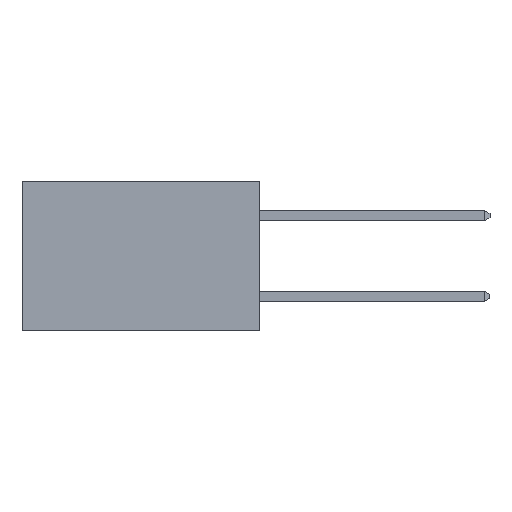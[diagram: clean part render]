
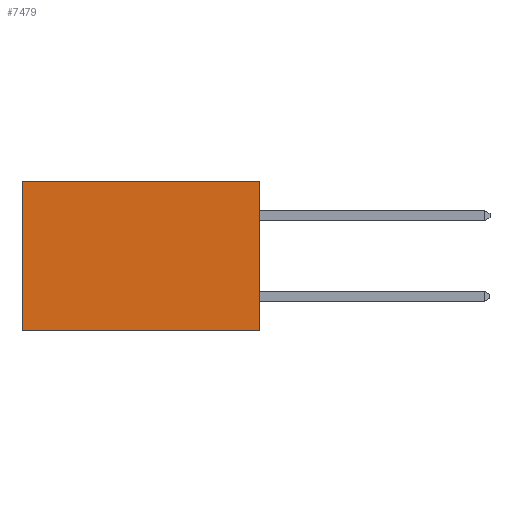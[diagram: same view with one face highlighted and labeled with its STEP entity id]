
A CAD part, left-side view. The second image highlights one B-rep face of the part: STEP entity #7479.
In plain terms, the highlighted planar face has unit normal (-1, 0, 0).
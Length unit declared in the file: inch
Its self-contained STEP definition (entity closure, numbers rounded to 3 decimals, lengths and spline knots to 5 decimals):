
#136 = CARTESIAN_POINT ( 'NONE',  ( 0.277, 0., 0. ) ) ;
#254 = EDGE_LOOP ( 'NONE', ( #7141, #4516, #5979, #3361 ) ) ;
#723 = LINE ( 'NONE', #136, #1090 ) ;
#1090 = VECTOR ( 'NONE', #7407, 39.37008 ) ;
#1256 = CARTESIAN_POINT ( 'NONE',  ( 0.277, 0.59, -0.37 ) ) ;
#1434 = CARTESIAN_POINT ( 'NONE',  ( 0.277, 0., -0.37 ) ) ;
#1784 = DIRECTION ( 'NONE',  ( 0., 0., -1. ) ) ;
#1935 = DIRECTION ( 'NONE',  ( 0., 0., -1. ) ) ;
#1947 = DIRECTION ( 'NONE',  ( 1., 0., 0. ) ) ;
#1956 = PLANE ( 'NONE',  #6717 ) ;
#1985 = CARTESIAN_POINT ( 'NONE',  ( 0.277, 0., -0.37 ) ) ;
#2057 = CARTESIAN_POINT ( 'NONE',  ( 0.277, 0.59, 0. ) ) ;
#2208 = CARTESIAN_POINT ( 'NONE',  ( 0.277, 0., -0.37 ) ) ;
#2312 = VERTEX_POINT ( 'NONE', #1256 ) ;
#2959 = VECTOR ( 'NONE', #3603, 39.37008 ) ;
#3147 = LINE ( 'NONE', #3537, #2959 ) ;
#3265 = EDGE_CURVE ( 'NONE', #3476, #2312, #3703, .T. ) ;
#3361 = ORIENTED_EDGE ( 'NONE', *, *, #6792, .T. ) ;
#3476 = VERTEX_POINT ( 'NONE', #1434 ) ;
#3481 = EDGE_CURVE ( 'NONE', #5042, #2312, #6556, .T. ) ;
#3537 = CARTESIAN_POINT ( 'NONE',  ( 0.277, 0., -0.37 ) ) ;
#3603 = DIRECTION ( 'NONE',  ( 0., 0., -1. ) ) ;
#3703 = LINE ( 'NONE', #2208, #5203 ) ;
#4220 = VERTEX_POINT ( 'NONE', #5339 ) ;
#4516 = ORIENTED_EDGE ( 'NONE', *, *, #3265, .F. ) ;
#4933 = FACE_OUTER_BOUND ( 'NONE', #254, .T. ) ;
#5042 = VERTEX_POINT ( 'NONE', #2057 ) ;
#5060 = CARTESIAN_POINT ( 'NONE',  ( 0.277, 0.59, -0.37 ) ) ;
#5106 = DIRECTION ( 'NONE',  ( 0., 1., 0. ) ) ;
#5112 = VECTOR ( 'NONE', #1784, 39.37008 ) ;
#5203 = VECTOR ( 'NONE', #5106, 39.37008 ) ;
#5339 = CARTESIAN_POINT ( 'NONE',  ( 0.277, 0., 0. ) ) ;
#5979 = ORIENTED_EDGE ( 'NONE', *, *, #7295, .F. ) ;
#6556 = LINE ( 'NONE', #5060, #5112 ) ;
#6717 = AXIS2_PLACEMENT_3D ( 'NONE', #1985, #1947, #1935 ) ;
#6792 = EDGE_CURVE ( 'NONE', #4220, #5042, #723, .T. ) ;
#7141 = ORIENTED_EDGE ( 'NONE', *, *, #3481, .T. ) ;
#7295 = EDGE_CURVE ( 'NONE', #4220, #3476, #3147, .T. ) ;
#7407 = DIRECTION ( 'NONE',  ( 0., 1., 0. ) ) ;
#7479 = ADVANCED_FACE ( 'NONE', ( #4933 ), #1956, .F. ) ;
